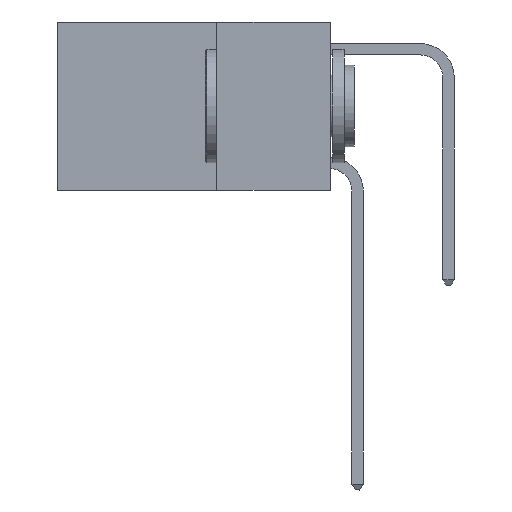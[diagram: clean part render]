
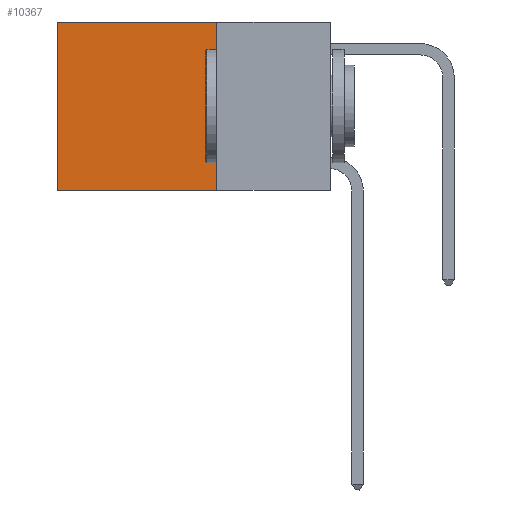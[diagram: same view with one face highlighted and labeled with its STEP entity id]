
A CAD part, left-side view. The second image highlights one B-rep face of the part: STEP entity #10367.
In plain terms, the highlighted planar face has unit normal (-1, 0, 0).
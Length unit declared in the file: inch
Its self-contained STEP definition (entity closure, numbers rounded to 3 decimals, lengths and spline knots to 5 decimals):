
#839 = CARTESIAN_POINT ( 'NONE',  ( 0.2625, 0.6, 0. ) ) ;
#907 = AXIS2_PLACEMENT_3D ( 'NONE', #2395, #10640, #7428 ) ;
#954 = CARTESIAN_POINT ( 'NONE',  ( 0.2625, 0.25, 0. ) ) ;
#1325 = VERTEX_POINT ( 'NONE', #3536 ) ;
#1605 = ORIENTED_EDGE ( 'NONE', *, *, #7599, .F. ) ;
#1642 = DIRECTION ( 'NONE',  ( 0., 1., 0. ) ) ;
#1879 = CARTESIAN_POINT ( 'NONE',  ( 0.2625, 0.6, 0. ) ) ;
#2095 = DIRECTION ( 'NONE',  ( 0., 0., -1. ) ) ;
#2257 = FACE_OUTER_BOUND ( 'NONE', #2435, .T. ) ;
#2395 = CARTESIAN_POINT ( 'NONE',  ( 0.2625, 0.25, 0. ) ) ;
#2435 = EDGE_LOOP ( 'NONE', ( #3702, #5025, #1605, #2903 ) ) ;
#2828 = CARTESIAN_POINT ( 'NONE',  ( 0.2625, 0.25, 0. ) ) ;
#2903 = ORIENTED_EDGE ( 'NONE', *, *, #5522, .T. ) ;
#3236 = VECTOR ( 'NONE', #2095, 39.37008 ) ;
#3311 = PLANE ( 'NONE',  #907 ) ;
#3497 = LINE ( 'NONE', #6670, #4143 ) ;
#3536 = CARTESIAN_POINT ( 'NONE',  ( 0.2625, 0.25, -0.37 ) ) ;
#3702 = ORIENTED_EDGE ( 'NONE', *, *, #8261, .T. ) ;
#3746 = VECTOR ( 'NONE', #10067, 39.37008 ) ;
#4143 = VECTOR ( 'NONE', #1642, 39.37008 ) ;
#4361 = LINE ( 'NONE', #1879, #7121 ) ;
#5025 = ORIENTED_EDGE ( 'NONE', *, *, #6207, .F. ) ;
#5522 = EDGE_CURVE ( 'NONE', #11320, #8239, #10560, .T. ) ;
#6207 = EDGE_CURVE ( 'NONE', #1325, #10272, #3497, .T. ) ;
#6670 = CARTESIAN_POINT ( 'NONE',  ( 0.2625, 0.25, -0.37 ) ) ;
#7121 = VECTOR ( 'NONE', #12367, 39.37008 ) ;
#7428 = DIRECTION ( 'NONE',  ( 0., 0., -1. ) ) ;
#7599 = EDGE_CURVE ( 'NONE', #11320, #1325, #12776, .T. ) ;
#7721 = CARTESIAN_POINT ( 'NONE',  ( 0.2625, 0.6, -0.37 ) ) ;
#8196 = CARTESIAN_POINT ( 'NONE',  ( 0.2625, 0.25, 0. ) ) ;
#8239 = VERTEX_POINT ( 'NONE', #839 ) ;
#8261 = EDGE_CURVE ( 'NONE', #8239, #10272, #4361, .T. ) ;
#10067 = DIRECTION ( 'NONE',  ( 0., 1., 0. ) ) ;
#10272 = VERTEX_POINT ( 'NONE', #7721 ) ;
#10367 = ADVANCED_FACE ( 'NONE', ( #2257 ), #3311, .F. ) ;
#10560 = LINE ( 'NONE', #2828, #3746 ) ;
#10640 = DIRECTION ( 'NONE',  ( 1., 0., 0. ) ) ;
#11320 = VERTEX_POINT ( 'NONE', #8196 ) ;
#12367 = DIRECTION ( 'NONE',  ( 0., 0., -1. ) ) ;
#12776 = LINE ( 'NONE', #954, #3236 ) ;
